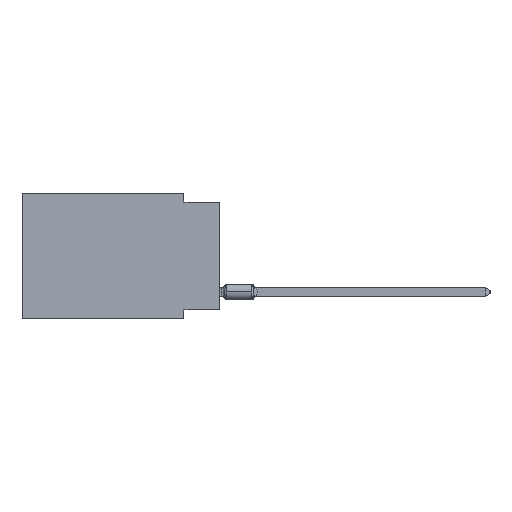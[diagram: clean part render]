
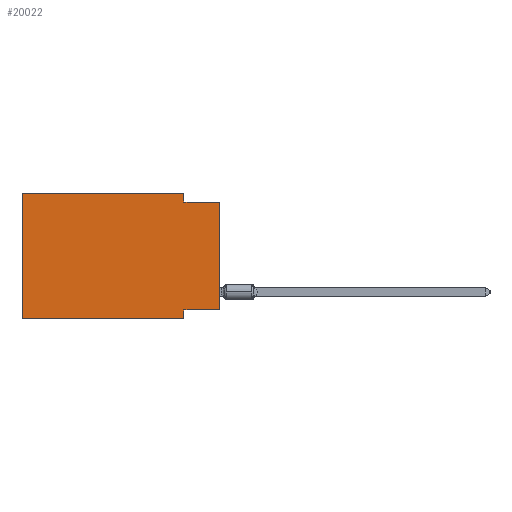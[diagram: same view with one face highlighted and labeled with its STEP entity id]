
A CAD part, left-side view. The second image highlights one B-rep face of the part: STEP entity #20022.
In plain terms, the highlighted planar face has unit normal (-1, 0, 0).
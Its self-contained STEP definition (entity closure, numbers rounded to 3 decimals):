
#326 = ORIENTED_EDGE ( 'NONE', *, *, #30591, .F. ) ;
#636 = FACE_OUTER_BOUND ( 'NONE', #34908, .T. ) ;
#1028 = EDGE_CURVE ( 'NONE', #17389, #14181, #38916, .T. ) ;
#2847 = VECTOR ( 'NONE', #25249, 1000. ) ;
#2860 = VERTEX_POINT ( 'NONE', #13942 ) ;
#3915 = VERTEX_POINT ( 'NONE', #29669 ) ;
#7546 = DIRECTION ( 'NONE',  ( 0., -1., 0. ) ) ;
#7749 = EDGE_CURVE ( 'NONE', #13013, #31983, #29420, .T. ) ;
#7955 = CARTESIAN_POINT ( 'NONE',  ( 0., 13.97, -8.89 ) ) ;
#8704 = CARTESIAN_POINT ( 'NONE',  ( 0., 2.54, -8.89 ) ) ;
#9001 = CARTESIAN_POINT ( 'NONE',  ( 0., 0., -0.635 ) ) ;
#9417 = LINE ( 'NONE', #37177, #33774 ) ;
#10409 = DIRECTION ( 'NONE',  ( 0., 0., -1. ) ) ;
#10591 = CARTESIAN_POINT ( 'NONE',  ( 0., 2.54, -8.89 ) ) ;
#10777 = DIRECTION ( 'NONE',  ( 1., 0., 0. ) ) ;
#10889 = LINE ( 'NONE', #31380, #38231 ) ;
#11077 = VECTOR ( 'NONE', #15541, 1000. ) ;
#11629 = EDGE_CURVE ( 'NONE', #3915, #17389, #9417, .T. ) ;
#11816 = CARTESIAN_POINT ( 'NONE',  ( 0., 0., 0. ) ) ;
#12020 = CARTESIAN_POINT ( 'NONE',  ( 0., 13.97, 0. ) ) ;
#12286 = ORIENTED_EDGE ( 'NONE', *, *, #1028, .F. ) ;
#13013 = VERTEX_POINT ( 'NONE', #24878 ) ;
#13445 = PLANE ( 'NONE',  #33908 ) ;
#13676 = ORIENTED_EDGE ( 'NONE', *, *, #11629, .F. ) ;
#13942 = CARTESIAN_POINT ( 'NONE',  ( 0., 2.54, 0. ) ) ;
#14181 = VERTEX_POINT ( 'NONE', #10591 ) ;
#14362 = VERTEX_POINT ( 'NONE', #9001 ) ;
#14391 = LINE ( 'NONE', #34667, #23810 ) ;
#14723 = CARTESIAN_POINT ( 'NONE',  ( 0., 2.54, -0.635 ) ) ;
#15541 = DIRECTION ( 'NONE',  ( 0., 0., 1. ) ) ;
#17389 = VERTEX_POINT ( 'NONE', #39447 ) ;
#18101 = LINE ( 'NONE', #40605, #36640 ) ;
#20022 = ADVANCED_FACE ( 'NONE', ( #636 ), #13445, .F. ) ;
#20799 = VECTOR ( 'NONE', #21865, 1000. ) ;
#21865 = DIRECTION ( 'NONE',  ( 0., -1., 0. ) ) ;
#23810 = VECTOR ( 'NONE', #7546, 1000. ) ;
#24111 = DIRECTION ( 'NONE',  ( 0., -1., 0. ) ) ;
#24817 = EDGE_CURVE ( 'NONE', #3915, #14362, #25902, .T. ) ;
#24878 = CARTESIAN_POINT ( 'NONE',  ( 0., 13.97, -8.89 ) ) ;
#25249 = DIRECTION ( 'NONE',  ( 0., 0., 1. ) ) ;
#25507 = EDGE_CURVE ( 'NONE', #2860, #41619, #18101, .T. ) ;
#25902 = LINE ( 'NONE', #11816, #2847 ) ;
#26868 = DIRECTION ( 'NONE',  ( 0., 0., -1. ) ) ;
#27520 = CARTESIAN_POINT ( 'NONE',  ( 0., 13.97, 0. ) ) ;
#27595 = LINE ( 'NONE', #7955, #20799 ) ;
#28994 = DIRECTION ( 'NONE',  ( 0., 0., -1. ) ) ;
#29400 = ORIENTED_EDGE ( 'NONE', *, *, #25507, .F. ) ;
#29420 = LINE ( 'NONE', #12020, #11077 ) ;
#29669 = CARTESIAN_POINT ( 'NONE',  ( 0., 0., -8.255 ) ) ;
#29704 = ORIENTED_EDGE ( 'NONE', *, *, #24817, .T. ) ;
#29709 = DIRECTION ( 'NONE',  ( 0., 1., 0. ) ) ;
#30582 = VECTOR ( 'NONE', #28994, 1000. ) ;
#30591 = EDGE_CURVE ( 'NONE', #41619, #14362, #10889, .T. ) ;
#31380 = CARTESIAN_POINT ( 'NONE',  ( 0., 0., -0.635 ) ) ;
#31958 = CARTESIAN_POINT ( 'NONE',  ( 0., 13.97, 0. ) ) ;
#31983 = VERTEX_POINT ( 'NONE', #31958 ) ;
#32251 = ORIENTED_EDGE ( 'NONE', *, *, #34469, .T. ) ;
#33774 = VECTOR ( 'NONE', #29709, 1000. ) ;
#33908 = AXIS2_PLACEMENT_3D ( 'NONE', #27520, #10777, #26868 ) ;
#34469 = EDGE_CURVE ( 'NONE', #13013, #14181, #27595, .T. ) ;
#34667 = CARTESIAN_POINT ( 'NONE',  ( 0., 13.97, 0. ) ) ;
#34908 = EDGE_LOOP ( 'NONE', ( #29704, #326, #29400, #37613, #35776, #32251, #12286, #13676 ) ) ;
#35776 = ORIENTED_EDGE ( 'NONE', *, *, #7749, .F. ) ;
#36640 = VECTOR ( 'NONE', #10409, 1000. ) ;
#37177 = CARTESIAN_POINT ( 'NONE',  ( 0., 0., -8.255 ) ) ;
#37613 = ORIENTED_EDGE ( 'NONE', *, *, #40639, .F. ) ;
#38231 = VECTOR ( 'NONE', #24111, 1000. ) ;
#38916 = LINE ( 'NONE', #8704, #30582 ) ;
#39447 = CARTESIAN_POINT ( 'NONE',  ( 0., 2.54, -8.255 ) ) ;
#40605 = CARTESIAN_POINT ( 'NONE',  ( 0., 2.54, 0. ) ) ;
#40639 = EDGE_CURVE ( 'NONE', #31983, #2860, #14391, .T. ) ;
#41619 = VERTEX_POINT ( 'NONE', #14723 ) ;
